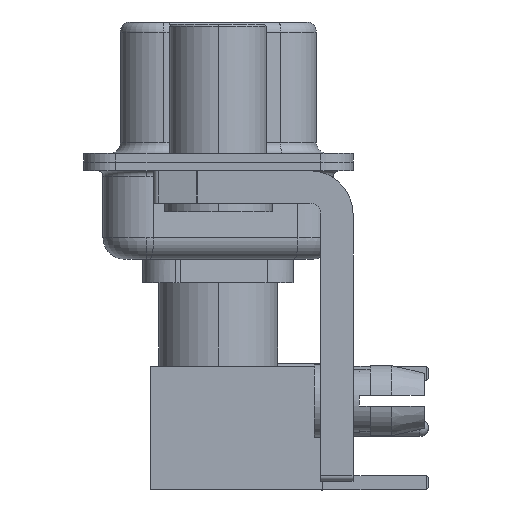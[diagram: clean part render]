
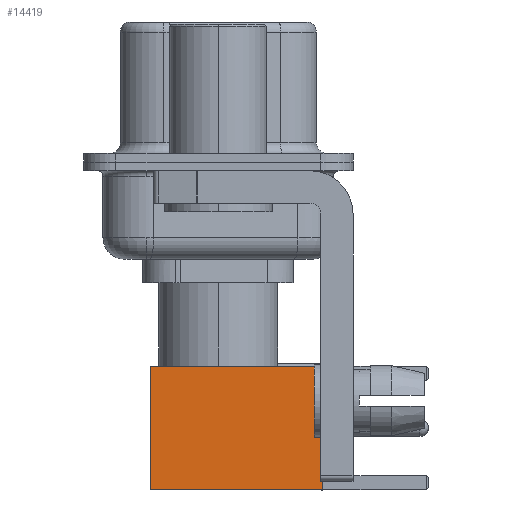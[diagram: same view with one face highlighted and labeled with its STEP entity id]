
A CAD part, left-side view. The second image highlights one B-rep face of the part: STEP entity #14419.
In plain terms, the highlighted face is planar.
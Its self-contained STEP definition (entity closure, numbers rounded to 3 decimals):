
#1447 = VERTEX_POINT ( 'NONE', #23420 ) ;
#1470 = ORIENTED_EDGE ( 'NONE', *, *, #26775, .T. ) ;
#4516 = DIRECTION ( 'NONE',  ( 0., 0., 1. ) ) ;
#4562 = DIRECTION ( 'NONE',  ( 0., 0., -1. ) ) ;
#5138 = DIRECTION ( 'NONE',  ( -1., 0., 0. ) ) ;
#5150 = VERTEX_POINT ( 'NONE', #22327 ) ;
#5535 = VECTOR ( 'NONE', #5138, 1000. ) ;
#7413 = CARTESIAN_POINT ( 'NONE',  ( 2.875, 2.875, 0. ) ) ;
#7687 = EDGE_LOOP ( 'NONE', ( #1470, #27093, #15734, #16201 ) ) ;
#7838 = DIRECTION ( 'NONE',  ( -1., 0., 0. ) ) ;
#9549 = DIRECTION ( 'NONE',  ( 0., 0., -1. ) ) ;
#10898 = CARTESIAN_POINT ( 'NONE',  ( 0., 2.875, 8. ) ) ;
#13077 = LINE ( 'NONE', #30739, #22303 ) ;
#14419 = ADVANCED_FACE ( 'NONE', ( #30650 ), #30313, .T. ) ;
#15734 = ORIENTED_EDGE ( 'NONE', *, *, #18680, .F. ) ;
#16201 = ORIENTED_EDGE ( 'NONE', *, *, #32609, .F. ) ;
#16308 = CARTESIAN_POINT ( 'NONE',  ( 2.875, 2.875, 0. ) ) ;
#16762 = EDGE_CURVE ( 'NONE', #29783, #5150, #13077, .T. ) ;
#17207 = CARTESIAN_POINT ( 'NONE',  ( 2.875, 2.875, 8. ) ) ;
#17403 = AXIS2_PLACEMENT_3D ( 'NONE', #7413, #27762, #4516 ) ;
#17522 = LINE ( 'NONE', #22779, #30288 ) ;
#18680 = EDGE_CURVE ( 'NONE', #1447, #5150, #27488, .T. ) ;
#22303 = VECTOR ( 'NONE', #7838, 1000. ) ;
#22327 = CARTESIAN_POINT ( 'NONE',  ( -2.875, 2.875, 0. ) ) ;
#22779 = CARTESIAN_POINT ( 'NONE',  ( 2.875, 2.875, 0. ) ) ;
#23420 = CARTESIAN_POINT ( 'NONE',  ( -2.875, 2.875, 8. ) ) ;
#24127 = VERTEX_POINT ( 'NONE', #17207 ) ;
#26775 = EDGE_CURVE ( 'NONE', #24127, #29783, #17522, .T. ) ;
#27093 = ORIENTED_EDGE ( 'NONE', *, *, #16762, .T. ) ;
#27488 = LINE ( 'NONE', #32594, #29449 ) ;
#27762 = DIRECTION ( 'NONE',  ( 0., 1., 0. ) ) ;
#28891 = LINE ( 'NONE', #10898, #5535 ) ;
#29449 = VECTOR ( 'NONE', #4562, 1000. ) ;
#29783 = VERTEX_POINT ( 'NONE', #16308 ) ;
#30288 = VECTOR ( 'NONE', #9549, 1000. ) ;
#30313 = PLANE ( 'NONE',  #17403 ) ;
#30650 = FACE_OUTER_BOUND ( 'NONE', #7687, .T. ) ;
#30739 = CARTESIAN_POINT ( 'NONE',  ( 0., 2.875, 0. ) ) ;
#32594 = CARTESIAN_POINT ( 'NONE',  ( -2.875, 2.875, 0. ) ) ;
#32609 = EDGE_CURVE ( 'NONE', #24127, #1447, #28891, .T. ) ;
